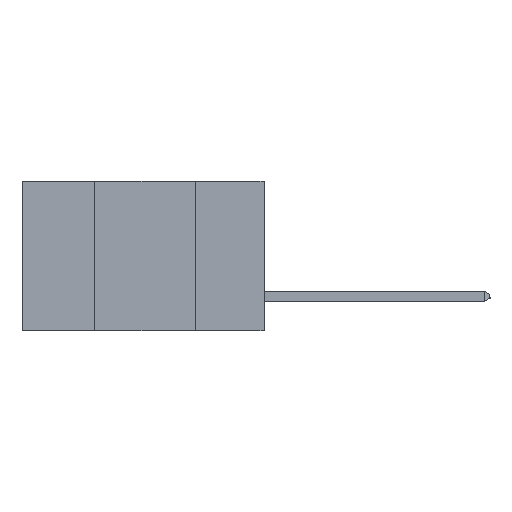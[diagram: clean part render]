
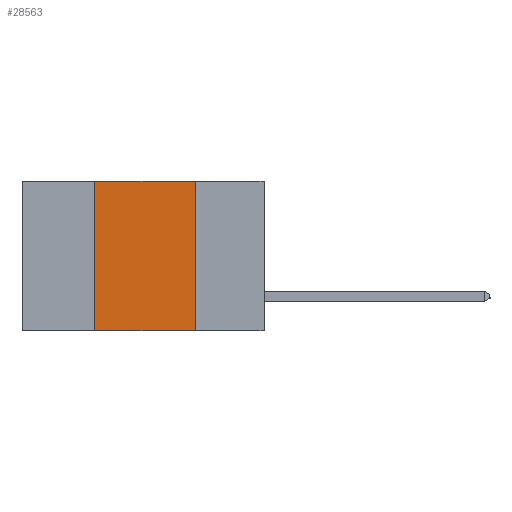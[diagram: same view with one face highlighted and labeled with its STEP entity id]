
A CAD part, left-side view. The second image highlights one B-rep face of the part: STEP entity #28563.
In plain terms, the highlighted planar face has unit normal (-1, 0, 0).
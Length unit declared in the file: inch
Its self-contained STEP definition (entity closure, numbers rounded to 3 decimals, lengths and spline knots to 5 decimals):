
#116 = DIRECTION ( 'NONE',  ( 0., 0., -1. ) ) ;
#724 = CARTESIAN_POINT ( 'NONE',  ( 0., 0.42, 0. ) ) ;
#1939 = VECTOR ( 'NONE', #23151, 39.37008 ) ;
#2889 = CARTESIAN_POINT ( 'NONE',  ( 0., 0.17, -0.37 ) ) ;
#3750 = VERTEX_POINT ( 'NONE', #25742 ) ;
#4068 = LINE ( 'NONE', #8436, #20448 ) ;
#5874 = VERTEX_POINT ( 'NONE', #8949 ) ;
#5902 = EDGE_CURVE ( 'NONE', #12510, #5874, #4068, .T. ) ;
#6642 = CARTESIAN_POINT ( 'NONE',  ( 0., 0.6, -0.37 ) ) ;
#6989 = DIRECTION ( 'NONE',  ( 1., 0., 0. ) ) ;
#8336 = ORIENTED_EDGE ( 'NONE', *, *, #19369, .F. ) ;
#8343 = DIRECTION ( 'NONE',  ( 0., -1., 0. ) ) ;
#8436 = CARTESIAN_POINT ( 'NONE',  ( 0., 0.6, 0. ) ) ;
#8949 = CARTESIAN_POINT ( 'NONE',  ( 0., 0.17, 0. ) ) ;
#9677 = FACE_OUTER_BOUND ( 'NONE', #17575, .T. ) ;
#10449 = ORIENTED_EDGE ( 'NONE', *, *, #17363, .T. ) ;
#11585 = LINE ( 'NONE', #6642, #16109 ) ;
#12039 = CARTESIAN_POINT ( 'NONE',  ( 0., 0.17, 0. ) ) ;
#12140 = DIRECTION ( 'NONE',  ( 0., 0., 1. ) ) ;
#12510 = VERTEX_POINT ( 'NONE', #12925 ) ;
#12925 = CARTESIAN_POINT ( 'NONE',  ( 0., 0.42, 0. ) ) ;
#13606 = ORIENTED_EDGE ( 'NONE', *, *, #19364, .F. ) ;
#13950 = LINE ( 'NONE', #724, #19086 ) ;
#16109 = VECTOR ( 'NONE', #22154, 39.37008 ) ;
#16377 = VERTEX_POINT ( 'NONE', #2889 ) ;
#17363 = EDGE_CURVE ( 'NONE', #3750, #16377, #11585, .T. ) ;
#17575 = EDGE_LOOP ( 'NONE', ( #13606, #25307, #8336, #10449 ) ) ;
#19086 = VECTOR ( 'NONE', #12140, 39.37008 ) ;
#19364 = EDGE_CURVE ( 'NONE', #5874, #16377, #25627, .T. ) ;
#19369 = EDGE_CURVE ( 'NONE', #3750, #12510, #13950, .T. ) ;
#20448 = VECTOR ( 'NONE', #8343, 39.37008 ) ;
#22154 = DIRECTION ( 'NONE',  ( 0., -1., 0. ) ) ;
#22385 = CARTESIAN_POINT ( 'NONE',  ( 0., 0.6, 0. ) ) ;
#23151 = DIRECTION ( 'NONE',  ( 0., 0., -1. ) ) ;
#24699 = PLANE ( 'NONE',  #24910 ) ;
#24910 = AXIS2_PLACEMENT_3D ( 'NONE', #22385, #6989, #116 ) ;
#25307 = ORIENTED_EDGE ( 'NONE', *, *, #5902, .F. ) ;
#25627 = LINE ( 'NONE', #12039, #1939 ) ;
#25742 = CARTESIAN_POINT ( 'NONE',  ( 0., 0.42, -0.37 ) ) ;
#28563 = ADVANCED_FACE ( 'NONE', ( #9677 ), #24699, .F. ) ;
